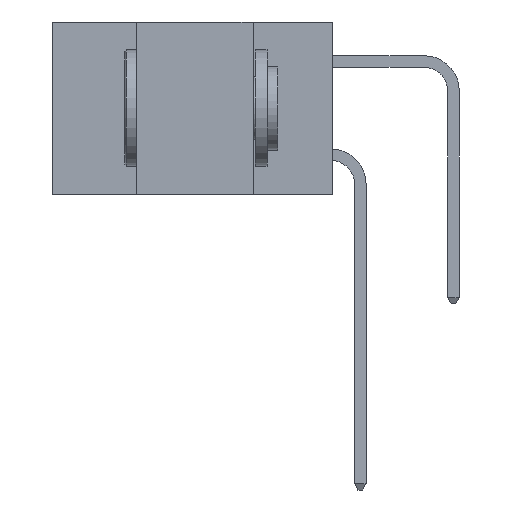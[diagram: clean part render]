
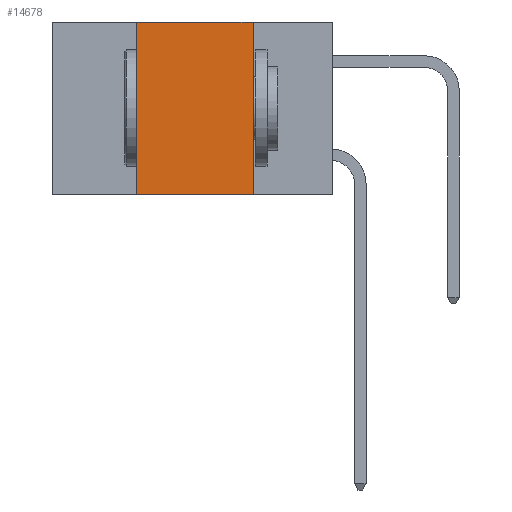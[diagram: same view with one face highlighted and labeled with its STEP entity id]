
A CAD part, left-side view. The second image highlights one B-rep face of the part: STEP entity #14678.
In plain terms, the highlighted planar face has unit normal (-1, 0, 0).
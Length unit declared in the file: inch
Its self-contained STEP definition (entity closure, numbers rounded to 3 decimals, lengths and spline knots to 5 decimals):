
#47 = CARTESIAN_POINT ( 'NONE',  ( 0., 0.6, 0. ) ) ;
#1404 = CARTESIAN_POINT ( 'NONE',  ( 0., 0.17, 0. ) ) ;
#1913 = ORIENTED_EDGE ( 'NONE', *, *, #6434, .F. ) ;
#1914 = CARTESIAN_POINT ( 'NONE',  ( 0., 0.42, -0.37 ) ) ;
#2531 = EDGE_CURVE ( 'NONE', #16946, #8832, #16708, .T. ) ;
#3071 = DIRECTION ( 'NONE',  ( 1., 0., 0. ) ) ;
#3545 = VECTOR ( 'NONE', #5251, 39.37008 ) ;
#5251 = DIRECTION ( 'NONE',  ( 0., -1., 0. ) ) ;
#5471 = EDGE_CURVE ( 'NONE', #8832, #15257, #17457, .T. ) ;
#6434 = EDGE_CURVE ( 'NONE', #15257, #7086, #13348, .T. ) ;
#6706 = ORIENTED_EDGE ( 'NONE', *, *, #17110, .T. ) ;
#7086 = VERTEX_POINT ( 'NONE', #12699 ) ;
#7276 = CARTESIAN_POINT ( 'NONE',  ( 0., 0.42, 0. ) ) ;
#7826 = LINE ( 'NONE', #13738, #3545 ) ;
#8832 = VERTEX_POINT ( 'NONE', #7276 ) ;
#9240 = VECTOR ( 'NONE', #15233, 39.37008 ) ;
#9988 = ORIENTED_EDGE ( 'NONE', *, *, #2531, .F. ) ;
#10149 = CARTESIAN_POINT ( 'NONE',  ( 0., 0.6, 0. ) ) ;
#11549 = PLANE ( 'NONE',  #13299 ) ;
#12699 = CARTESIAN_POINT ( 'NONE',  ( 0., 0.17, -0.37 ) ) ;
#12903 = VECTOR ( 'NONE', #18056, 39.37008 ) ;
#13022 = DIRECTION ( 'NONE',  ( 0., 0., -1. ) ) ;
#13299 = AXIS2_PLACEMENT_3D ( 'NONE', #10149, #3071, #13022 ) ;
#13336 = ORIENTED_EDGE ( 'NONE', *, *, #5471, .F. ) ;
#13348 = LINE ( 'NONE', #18051, #12903 ) ;
#13452 = EDGE_LOOP ( 'NONE', ( #1913, #13336, #9988, #6706 ) ) ;
#13738 = CARTESIAN_POINT ( 'NONE',  ( 0., 0.6, -0.37 ) ) ;
#14678 = ADVANCED_FACE ( 'NONE', ( #17481 ), #11549, .F. ) ;
#15233 = DIRECTION ( 'NONE',  ( 0., 0., 1. ) ) ;
#15257 = VERTEX_POINT ( 'NONE', #1404 ) ;
#15732 = CARTESIAN_POINT ( 'NONE',  ( 0., 0.42, -0.37 ) ) ;
#16708 = LINE ( 'NONE', #15732, #9240 ) ;
#16946 = VERTEX_POINT ( 'NONE', #1914 ) ;
#17043 = DIRECTION ( 'NONE',  ( 0., -1., 0. ) ) ;
#17052 = VECTOR ( 'NONE', #17043, 39.37008 ) ;
#17110 = EDGE_CURVE ( 'NONE', #16946, #7086, #7826, .T. ) ;
#17457 = LINE ( 'NONE', #47, #17052 ) ;
#17481 = FACE_OUTER_BOUND ( 'NONE', #13452, .T. ) ;
#18051 = CARTESIAN_POINT ( 'NONE',  ( 0., 0.17, -0.37 ) ) ;
#18056 = DIRECTION ( 'NONE',  ( 0., 0., -1. ) ) ;
